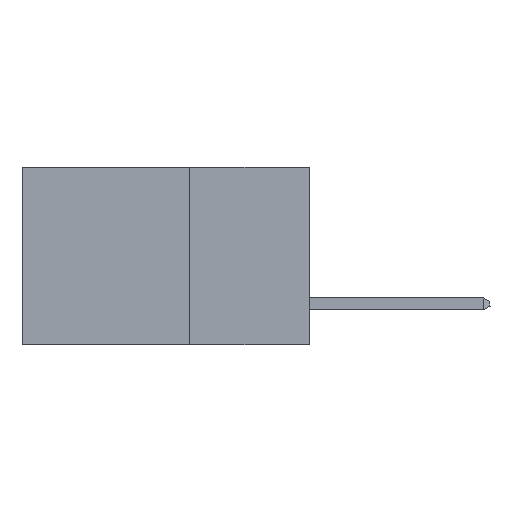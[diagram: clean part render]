
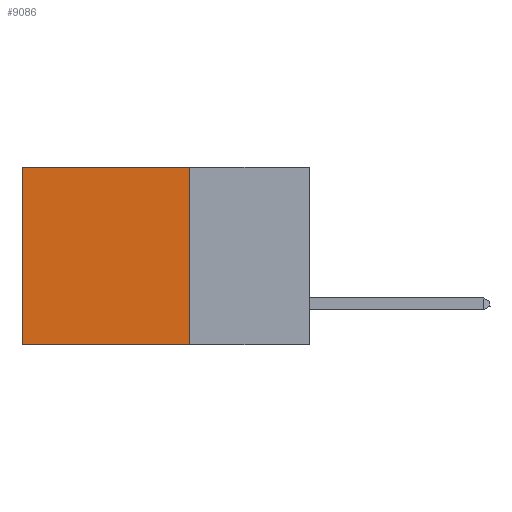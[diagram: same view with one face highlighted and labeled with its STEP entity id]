
A CAD part, left-side view. The second image highlights one B-rep face of the part: STEP entity #9086.
In plain terms, the highlighted planar face has unit normal (-1, 0, 0).
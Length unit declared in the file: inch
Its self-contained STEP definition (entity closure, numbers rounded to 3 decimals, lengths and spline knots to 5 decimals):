
#97 = LINE ( 'NONE', #2664, #1800 ) ;
#335 = ORIENTED_EDGE ( 'NONE', *, *, #6890, .T. ) ;
#1272 = LINE ( 'NONE', #10766, #10700 ) ;
#1564 = CARTESIAN_POINT ( 'NONE',  ( 0.2875, 0.6, -0.37 ) ) ;
#1800 = VECTOR ( 'NONE', #11813, 39.37008 ) ;
#1893 = FACE_OUTER_BOUND ( 'NONE', #5853, .T. ) ;
#1976 = VERTEX_POINT ( 'NONE', #1564 ) ;
#2244 = DIRECTION ( 'NONE',  ( 1., 0., 0. ) ) ;
#2496 = ORIENTED_EDGE ( 'NONE', *, *, #5971, .F. ) ;
#2664 = CARTESIAN_POINT ( 'NONE',  ( 0.2875, 0.25, 0. ) ) ;
#2768 = VERTEX_POINT ( 'NONE', #5625 ) ;
#3404 = DIRECTION ( 'NONE',  ( 0., 1., 0. ) ) ;
#3497 = LINE ( 'NONE', #11340, #5207 ) ;
#4041 = EDGE_CURVE ( 'NONE', #2768, #1976, #10184, .T. ) ;
#4052 = CARTESIAN_POINT ( 'NONE',  ( 0.2875, 0.6, 0. ) ) ;
#5207 = VECTOR ( 'NONE', #8578, 39.37008 ) ;
#5625 = CARTESIAN_POINT ( 'NONE',  ( 0.2875, 0.6, 0. ) ) ;
#5853 = EDGE_LOOP ( 'NONE', ( #8984, #2496, #8570, #335 ) ) ;
#5915 = DIRECTION ( 'NONE',  ( 0., 0., -1. ) ) ;
#5971 = EDGE_CURVE ( 'NONE', #9879, #1976, #1272, .T. ) ;
#6394 = EDGE_CURVE ( 'NONE', #7925, #9879, #97, .T. ) ;
#6890 = EDGE_CURVE ( 'NONE', #7925, #2768, #3497, .T. ) ;
#7309 = CARTESIAN_POINT ( 'NONE',  ( 0.2875, 0.25, -0.37 ) ) ;
#7925 = VERTEX_POINT ( 'NONE', #10679 ) ;
#8108 = AXIS2_PLACEMENT_3D ( 'NONE', #10432, #2244, #10591 ) ;
#8570 = ORIENTED_EDGE ( 'NONE', *, *, #6394, .F. ) ;
#8578 = DIRECTION ( 'NONE',  ( 0., 1., 0. ) ) ;
#8984 = ORIENTED_EDGE ( 'NONE', *, *, #4041, .T. ) ;
#9086 = ADVANCED_FACE ( 'NONE', ( #1893 ), #9492, .F. ) ;
#9492 = PLANE ( 'NONE',  #8108 ) ;
#9778 = VECTOR ( 'NONE', #5915, 39.37008 ) ;
#9879 = VERTEX_POINT ( 'NONE', #7309 ) ;
#10184 = LINE ( 'NONE', #4052, #9778 ) ;
#10432 = CARTESIAN_POINT ( 'NONE',  ( 0.2875, 0.25, 0. ) ) ;
#10591 = DIRECTION ( 'NONE',  ( 0., 0., -1. ) ) ;
#10679 = CARTESIAN_POINT ( 'NONE',  ( 0.2875, 0.25, 0. ) ) ;
#10700 = VECTOR ( 'NONE', #3404, 39.37008 ) ;
#10766 = CARTESIAN_POINT ( 'NONE',  ( 0.2875, 0.25, -0.37 ) ) ;
#11340 = CARTESIAN_POINT ( 'NONE',  ( 0.2875, 0.25, 0. ) ) ;
#11813 = DIRECTION ( 'NONE',  ( 0., 0., -1. ) ) ;
